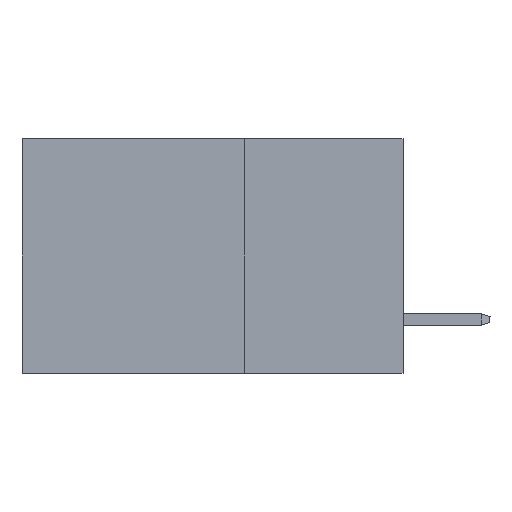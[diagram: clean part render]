
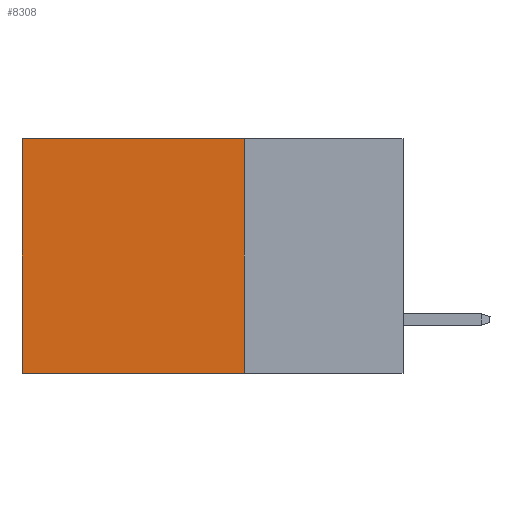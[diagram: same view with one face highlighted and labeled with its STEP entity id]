
A CAD part, left-side view. The second image highlights one B-rep face of the part: STEP entity #8308.
In plain terms, the highlighted planar face has unit normal (-1, 0, 0).
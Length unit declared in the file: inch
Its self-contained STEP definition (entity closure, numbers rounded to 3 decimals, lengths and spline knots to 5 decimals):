
#180 = CARTESIAN_POINT ( 'NONE',  ( 0.2875, 0.6, 0. ) ) ;
#886 = DIRECTION ( 'NONE',  ( 0., 0., -1. ) ) ;
#1331 = LINE ( 'NONE', #8179, #8039 ) ;
#1417 = ORIENTED_EDGE ( 'NONE', *, *, #12170, .T. ) ;
#1450 = DIRECTION ( 'NONE',  ( 0., 0., -1. ) ) ;
#1570 = VECTOR ( 'NONE', #7730, 39.37008 ) ;
#1717 = EDGE_CURVE ( 'NONE', #3730, #8593, #9621, .T. ) ;
#2527 = EDGE_CURVE ( 'NONE', #10322, #8593, #11252, .T. ) ;
#2760 = PLANE ( 'NONE',  #10645 ) ;
#2842 = CARTESIAN_POINT ( 'NONE',  ( 0.2875, 0.25, 0. ) ) ;
#3730 = VERTEX_POINT ( 'NONE', #180 ) ;
#4619 = VECTOR ( 'NONE', #1450, 39.37008 ) ;
#5056 = VECTOR ( 'NONE', #8343, 39.37008 ) ;
#5530 = FACE_OUTER_BOUND ( 'NONE', #10785, .T. ) ;
#7166 = DIRECTION ( 'NONE',  ( 0., 1., 0. ) ) ;
#7542 = CARTESIAN_POINT ( 'NONE',  ( 0.2875, 0.6, 0. ) ) ;
#7730 = DIRECTION ( 'NONE',  ( 0., 0., -1. ) ) ;
#7842 = CARTESIAN_POINT ( 'NONE',  ( 0.2875, 0.6, -0.37 ) ) ;
#7998 = ORIENTED_EDGE ( 'NONE', *, *, #2527, .F. ) ;
#8039 = VECTOR ( 'NONE', #7166, 39.37008 ) ;
#8104 = CARTESIAN_POINT ( 'NONE',  ( 0.2875, 0.25, 0. ) ) ;
#8159 = CARTESIAN_POINT ( 'NONE',  ( 0.2875, 0.25, -0.37 ) ) ;
#8179 = CARTESIAN_POINT ( 'NONE',  ( 0.2875, 0.25, 0. ) ) ;
#8308 = ADVANCED_FACE ( 'NONE', ( #5530 ), #2760, .F. ) ;
#8343 = DIRECTION ( 'NONE',  ( 0., 1., 0. ) ) ;
#8593 = VERTEX_POINT ( 'NONE', #7842 ) ;
#9289 = CARTESIAN_POINT ( 'NONE',  ( 0.2875, 0.25, -0.37 ) ) ;
#9621 = LINE ( 'NONE', #7542, #1570 ) ;
#10322 = VERTEX_POINT ( 'NONE', #8159 ) ;
#10645 = AXIS2_PLACEMENT_3D ( 'NONE', #2842, #12323, #886 ) ;
#10731 = CARTESIAN_POINT ( 'NONE',  ( 0.2875, 0.25, 0. ) ) ;
#10785 = EDGE_LOOP ( 'NONE', ( #12053, #7998, #11089, #1417 ) ) ;
#11078 = LINE ( 'NONE', #8104, #4619 ) ;
#11089 = ORIENTED_EDGE ( 'NONE', *, *, #11565, .F. ) ;
#11252 = LINE ( 'NONE', #9289, #5056 ) ;
#11565 = EDGE_CURVE ( 'NONE', #12347, #10322, #11078, .T. ) ;
#12053 = ORIENTED_EDGE ( 'NONE', *, *, #1717, .T. ) ;
#12170 = EDGE_CURVE ( 'NONE', #12347, #3730, #1331, .T. ) ;
#12323 = DIRECTION ( 'NONE',  ( 1., 0., 0. ) ) ;
#12347 = VERTEX_POINT ( 'NONE', #10731 ) ;
